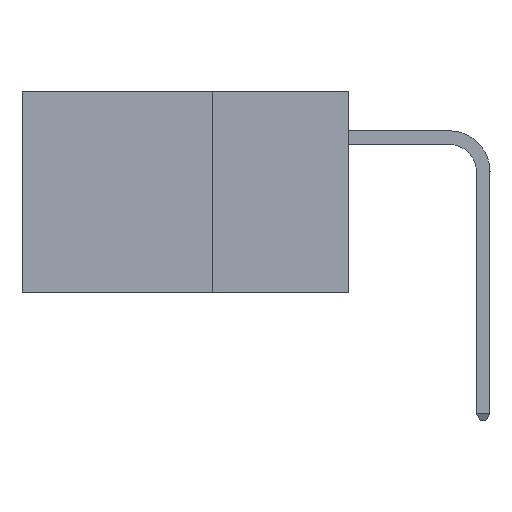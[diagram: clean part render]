
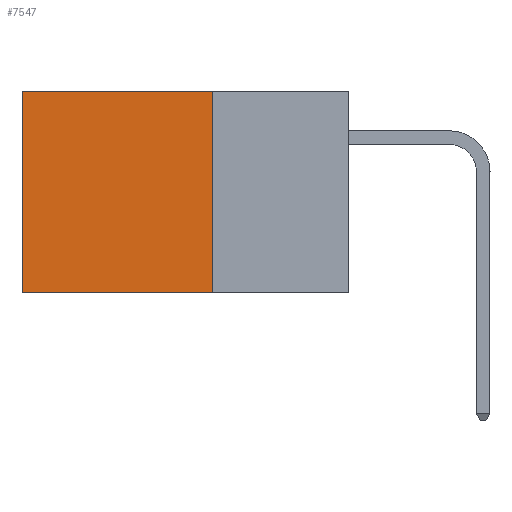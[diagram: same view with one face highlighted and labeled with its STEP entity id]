
A CAD part, left-side view. The second image highlights one B-rep face of the part: STEP entity #7547.
In plain terms, the highlighted planar face has unit normal (-1, 0, 0).
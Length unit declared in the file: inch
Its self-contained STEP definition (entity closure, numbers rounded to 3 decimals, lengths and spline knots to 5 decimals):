
#1219 = DIRECTION ( 'NONE',  ( 0., 0., -1. ) ) ;
#1350 = EDGE_CURVE ( 'NONE', #3665, #4180, #5131, .T. ) ;
#3340 = EDGE_CURVE ( 'NONE', #3665, #18474, #17281, .T. ) ;
#3402 = DIRECTION ( 'NONE',  ( 1., 0., 0. ) ) ;
#3665 = VERTEX_POINT ( 'NONE', #21778 ) ;
#3911 = ORIENTED_EDGE ( 'NONE', *, *, #1350, .T. ) ;
#4180 = VERTEX_POINT ( 'NONE', #5036 ) ;
#5036 = CARTESIAN_POINT ( 'NONE',  ( 0.2875, 0.6, 0. ) ) ;
#5131 = LINE ( 'NONE', #23906, #14117 ) ;
#5257 = DIRECTION ( 'NONE',  ( 0., 1., 0. ) ) ;
#5578 = CARTESIAN_POINT ( 'NONE',  ( 0.2875, 0.25, -0.37 ) ) ;
#5829 = LINE ( 'NONE', #7409, #9484 ) ;
#7409 = CARTESIAN_POINT ( 'NONE',  ( 0.2875, 0.6, 0. ) ) ;
#7547 = ADVANCED_FACE ( 'NONE', ( #21937 ), #16325, .F. ) ;
#9484 = VECTOR ( 'NONE', #11190, 39.37008 ) ;
#10821 = EDGE_LOOP ( 'NONE', ( #11781, #23975, #14584, #3911 ) ) ;
#10857 = VERTEX_POINT ( 'NONE', #13392 ) ;
#11190 = DIRECTION ( 'NONE',  ( 0., 0., -1. ) ) ;
#11781 = ORIENTED_EDGE ( 'NONE', *, *, #21811, .T. ) ;
#11894 = DIRECTION ( 'NONE',  ( 0., 1., 0. ) ) ;
#13274 = VECTOR ( 'NONE', #11894, 39.37008 ) ;
#13392 = CARTESIAN_POINT ( 'NONE',  ( 0.2875, 0.6, -0.37 ) ) ;
#13623 = CARTESIAN_POINT ( 'NONE',  ( 0.2875, 0.25, 0. ) ) ;
#14117 = VECTOR ( 'NONE', #5257, 39.37008 ) ;
#14584 = ORIENTED_EDGE ( 'NONE', *, *, #3340, .F. ) ;
#16037 = LINE ( 'NONE', #23227, #13274 ) ;
#16325 = PLANE ( 'NONE',  #20394 ) ;
#17281 = LINE ( 'NONE', #13623, #19371 ) ;
#18474 = VERTEX_POINT ( 'NONE', #5578 ) ;
#18799 = EDGE_CURVE ( 'NONE', #18474, #10857, #16037, .T. ) ;
#19371 = VECTOR ( 'NONE', #23003, 39.37008 ) ;
#20229 = CARTESIAN_POINT ( 'NONE',  ( 0.2875, 0.25, 0. ) ) ;
#20394 = AXIS2_PLACEMENT_3D ( 'NONE', #20229, #3402, #1219 ) ;
#21778 = CARTESIAN_POINT ( 'NONE',  ( 0.2875, 0.25, 0. ) ) ;
#21811 = EDGE_CURVE ( 'NONE', #4180, #10857, #5829, .T. ) ;
#21937 = FACE_OUTER_BOUND ( 'NONE', #10821, .T. ) ;
#23003 = DIRECTION ( 'NONE',  ( 0., 0., -1. ) ) ;
#23227 = CARTESIAN_POINT ( 'NONE',  ( 0.2875, 0.25, -0.37 ) ) ;
#23906 = CARTESIAN_POINT ( 'NONE',  ( 0.2875, 0.25, 0. ) ) ;
#23975 = ORIENTED_EDGE ( 'NONE', *, *, #18799, .F. ) ;
